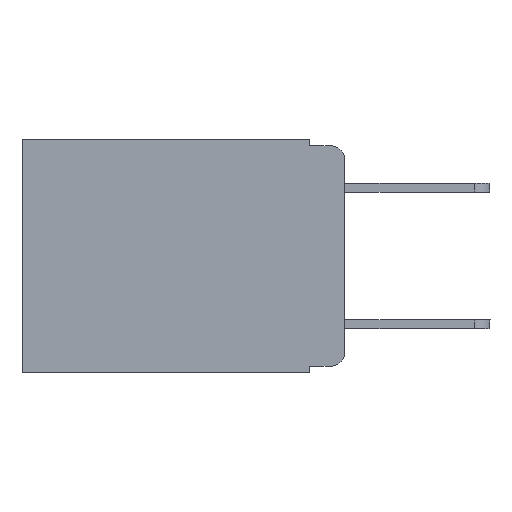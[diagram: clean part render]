
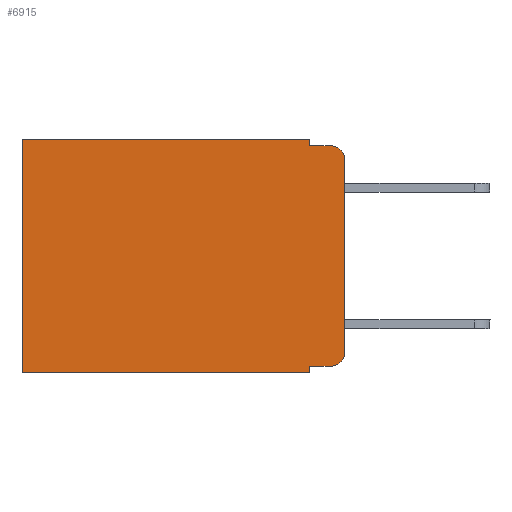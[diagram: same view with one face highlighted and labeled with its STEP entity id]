
A CAD part, left-side view. The second image highlights one B-rep face of the part: STEP entity #6915.
In plain terms, the highlighted planar face has unit normal (-1, 0, 0).
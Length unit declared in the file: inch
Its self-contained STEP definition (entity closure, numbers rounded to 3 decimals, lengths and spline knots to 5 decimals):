
#55 = ORIENTED_EDGE ( 'NONE', *, *, #9980, .T. ) ;
#56 = DIRECTION ( 'NONE',  ( 1., 0., 0. ) ) ;
#81 = ORIENTED_EDGE ( 'NONE', *, *, #4301, .F. ) ;
#194 = LINE ( 'NONE', #3794, #642 ) ;
#334 = CARTESIAN_POINT ( 'NONE',  ( 0.298, 0.051, 0. ) ) ;
#581 = DIRECTION ( 'NONE',  ( 0., 0., -1. ) ) ;
#642 = VECTOR ( 'NONE', #4656, 39.37008 ) ;
#772 = DIRECTION ( 'NONE',  ( 0., 0., -1. ) ) ;
#859 = ORIENTED_EDGE ( 'NONE', *, *, #4549, .F. ) ;
#1255 = CARTESIAN_POINT ( 'NONE',  ( 0.298, 0.02, -0.03 ) ) ;
#1284 = VERTEX_POINT ( 'NONE', #8225 ) ;
#1363 = DIRECTION ( 'NONE',  ( -1., 0., 0. ) ) ;
#1758 = CARTESIAN_POINT ( 'NONE',  ( 0.298, 0.051, -0.01 ) ) ;
#1772 = CARTESIAN_POINT ( 'NONE',  ( 0.298, 0.051, 0. ) ) ;
#1801 = VERTEX_POINT ( 'NONE', #3017 ) ;
#1846 = LINE ( 'NONE', #6178, #8324 ) ;
#1971 = PLANE ( 'NONE',  #11193 ) ;
#2161 = CARTESIAN_POINT ( 'NONE',  ( 0.298, 0.473, 0. ) ) ;
#2429 = VERTEX_POINT ( 'NONE', #10418 ) ;
#2496 = VERTEX_POINT ( 'NONE', #6619 ) ;
#2770 = DIRECTION ( 'NONE',  ( 0., 1., 0. ) ) ;
#3017 = CARTESIAN_POINT ( 'NONE',  ( 0.298, 0.051, -0.333 ) ) ;
#3304 = VERTEX_POINT ( 'NONE', #2161 ) ;
#3351 = DIRECTION ( 'NONE',  ( 0., 0., -1. ) ) ;
#3578 = EDGE_CURVE ( 'NONE', #3304, #2429, #8357, .T. ) ;
#3794 = CARTESIAN_POINT ( 'NONE',  ( 0.298, 0.051, -0.333 ) ) ;
#3818 = LINE ( 'NONE', #5738, #5632 ) ;
#4022 = CARTESIAN_POINT ( 'NONE',  ( 0.298, 0., 0. ) ) ;
#4137 = EDGE_CURVE ( 'NONE', #4388, #2496, #6561, .T. ) ;
#4301 = EDGE_CURVE ( 'NONE', #5993, #1284, #5653, .T. ) ;
#4330 = ORIENTED_EDGE ( 'NONE', *, *, #5739, .T. ) ;
#4388 = VERTEX_POINT ( 'NONE', #5749 ) ;
#4460 = LINE ( 'NONE', #10398, #7746 ) ;
#4479 = CARTESIAN_POINT ( 'NONE',  ( 0.298, 0., 0. ) ) ;
#4513 = DIRECTION ( 'NONE',  ( 0., 0., -1. ) ) ;
#4549 = EDGE_CURVE ( 'NONE', #1801, #4925, #11854, .T. ) ;
#4656 = DIRECTION ( 'NONE',  ( 0., -1., 0. ) ) ;
#4925 = VERTEX_POINT ( 'NONE', #6024 ) ;
#4971 = AXIS2_PLACEMENT_3D ( 'NONE', #7179, #1363, #3351 ) ;
#5384 = ORIENTED_EDGE ( 'NONE', *, *, #10902, .F. ) ;
#5418 = EDGE_CURVE ( 'NONE', #9491, #1284, #7429, .T. ) ;
#5494 = VECTOR ( 'NONE', #7122, 39.37008 ) ;
#5541 = ORIENTED_EDGE ( 'NONE', *, *, #5418, .T. ) ;
#5632 = VECTOR ( 'NONE', #2770, 39.37008 ) ;
#5653 = LINE ( 'NONE', #1758, #10177 ) ;
#5738 = CARTESIAN_POINT ( 'NONE',  ( 0.298, 0., 0. ) ) ;
#5739 = EDGE_CURVE ( 'NONE', #12471, #3304, #3818, .T. ) ;
#5749 = CARTESIAN_POINT ( 'NONE',  ( 0.298, 0.02, -0.333 ) ) ;
#5894 = FACE_OUTER_BOUND ( 'NONE', #9209, .T. ) ;
#5993 = VERTEX_POINT ( 'NONE', #7887 ) ;
#6024 = CARTESIAN_POINT ( 'NONE',  ( 0.298, 0.051, -0.343 ) ) ;
#6037 = DIRECTION ( 'NONE',  ( -1., 0., 0. ) ) ;
#6176 = CARTESIAN_POINT ( 'NONE',  ( 0.298, 0., -0.03 ) ) ;
#6178 = CARTESIAN_POINT ( 'NONE',  ( 0.298, 0., -0.343 ) ) ;
#6561 = CIRCLE ( 'NONE', #4971, 0.02 ) ;
#6619 = CARTESIAN_POINT ( 'NONE',  ( 0.298, 0., -0.313 ) ) ;
#6915 = ADVANCED_FACE ( 'NONE', ( #5894 ), #1971, .F. ) ;
#6921 = LINE ( 'NONE', #4479, #11751 ) ;
#7122 = DIRECTION ( 'NONE',  ( 0., 0., -1. ) ) ;
#7179 = CARTESIAN_POINT ( 'NONE',  ( 0.298, 0.02, -0.313 ) ) ;
#7429 = CIRCLE ( 'NONE', #11996, 0.02 ) ;
#7697 = ORIENTED_EDGE ( 'NONE', *, *, #7785, .F. ) ;
#7746 = VECTOR ( 'NONE', #772, 39.37008 ) ;
#7785 = EDGE_CURVE ( 'NONE', #9491, #2496, #6921, .T. ) ;
#7821 = ORIENTED_EDGE ( 'NONE', *, *, #3578, .T. ) ;
#7887 = CARTESIAN_POINT ( 'NONE',  ( 0.298, 0.051, -0.01 ) ) ;
#8225 = CARTESIAN_POINT ( 'NONE',  ( 0.298, 0.02, -0.01 ) ) ;
#8324 = VECTOR ( 'NONE', #10987, 39.37008 ) ;
#8357 = LINE ( 'NONE', #11316, #10650 ) ;
#8502 = DIRECTION ( 'NONE',  ( 0., -1., 0. ) ) ;
#8676 = DIRECTION ( 'NONE',  ( 0., 0., -1. ) ) ;
#9209 = EDGE_LOOP ( 'NONE', ( #7697, #5541, #81, #10228, #4330, #7821, #5384, #859, #55, #10851 ) ) ;
#9491 = VERTEX_POINT ( 'NONE', #6176 ) ;
#9980 = EDGE_CURVE ( 'NONE', #1801, #4388, #194, .T. ) ;
#10177 = VECTOR ( 'NONE', #8502, 39.37008 ) ;
#10228 = ORIENTED_EDGE ( 'NONE', *, *, #10703, .F. ) ;
#10398 = CARTESIAN_POINT ( 'NONE',  ( 0.298, 0.051, 0. ) ) ;
#10418 = CARTESIAN_POINT ( 'NONE',  ( 0.298, 0.473, -0.343 ) ) ;
#10650 = VECTOR ( 'NONE', #4513, 39.37008 ) ;
#10703 = EDGE_CURVE ( 'NONE', #12471, #5993, #4460, .T. ) ;
#10757 = DIRECTION ( 'NONE',  ( 0., 0., -1. ) ) ;
#10851 = ORIENTED_EDGE ( 'NONE', *, *, #4137, .T. ) ;
#10902 = EDGE_CURVE ( 'NONE', #4925, #2429, #1846, .T. ) ;
#10987 = DIRECTION ( 'NONE',  ( 0., 1., 0. ) ) ;
#11193 = AXIS2_PLACEMENT_3D ( 'NONE', #4022, #56, #8676 ) ;
#11316 = CARTESIAN_POINT ( 'NONE',  ( 0.298, 0.473, 0. ) ) ;
#11751 = VECTOR ( 'NONE', #581, 39.37008 ) ;
#11854 = LINE ( 'NONE', #334, #5494 ) ;
#11996 = AXIS2_PLACEMENT_3D ( 'NONE', #1255, #6037, #10757 ) ;
#12471 = VERTEX_POINT ( 'NONE', #1772 ) ;
